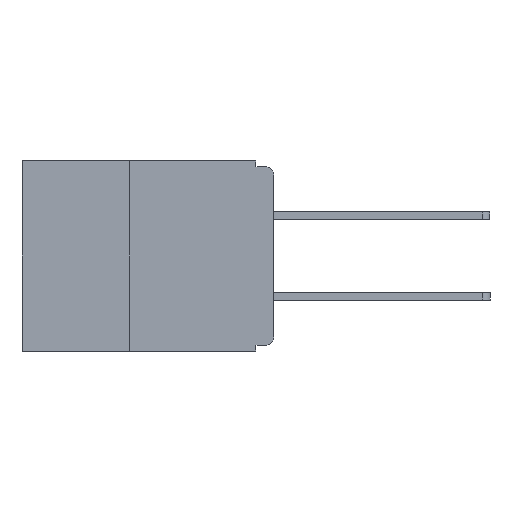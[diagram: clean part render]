
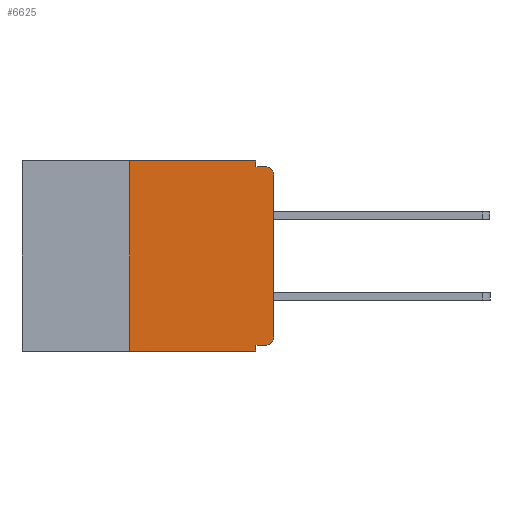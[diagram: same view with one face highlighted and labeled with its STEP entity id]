
A CAD part, left-side view. The second image highlights one B-rep face of the part: STEP entity #6625.
In plain terms, the highlighted planar face has unit normal (-1, 0, 0).
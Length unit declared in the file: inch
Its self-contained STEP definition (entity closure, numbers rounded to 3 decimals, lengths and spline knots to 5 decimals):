
#55 = VERTEX_POINT ( 'NONE', #28646 ) ;
#768 = CIRCLE ( 'NONE', #29298, 0.015 ) ;
#797 = VERTEX_POINT ( 'NONE', #12982 ) ;
#1027 = VERTEX_POINT ( 'NONE', #7774 ) ;
#1044 = CARTESIAN_POINT ( 'NONE',  ( 0., 0., -0.305 ) ) ;
#1522 = VERTEX_POINT ( 'NONE', #11934 ) ;
#2171 = ORIENTED_EDGE ( 'NONE', *, *, #8402, .F. ) ;
#2189 = EDGE_CURVE ( 'NONE', #13385, #2353, #28413, .T. ) ;
#2353 = VERTEX_POINT ( 'NONE', #18320 ) ;
#2566 = EDGE_CURVE ( 'NONE', #1027, #2353, #13446, .T. ) ;
#2572 = CARTESIAN_POINT ( 'NONE',  ( 0., 0.031, 0. ) ) ;
#3139 = CARTESIAN_POINT ( 'NONE',  ( 0., 0.437, 0. ) ) ;
#3473 = VECTOR ( 'NONE', #23259, 39.37008 ) ;
#3894 = ORIENTED_EDGE ( 'NONE', *, *, #29182, .F. ) ;
#4364 = CARTESIAN_POINT ( 'NONE',  ( 0., 0.437, -0.33 ) ) ;
#4496 = DIRECTION ( 'NONE',  ( 0., -1., 0. ) ) ;
#5229 = EDGE_CURVE ( 'NONE', #1522, #14036, #5631, .T. ) ;
#5631 = LINE ( 'NONE', #3139, #28974 ) ;
#6399 = EDGE_CURVE ( 'NONE', #1027, #1522, #10724, .T. ) ;
#6476 = DIRECTION ( 'NONE',  ( -1., 0., 0. ) ) ;
#6625 = ADVANCED_FACE ( 'NONE', ( #10335 ), #24892, .F. ) ;
#6678 = CARTESIAN_POINT ( 'NONE',  ( 0., 0.031, 0. ) ) ;
#7363 = EDGE_LOOP ( 'NONE', ( #29333, #20917, #2171, #3894, #30257, #23526, #18733, #17245, #11721, #22951 ) ) ;
#7774 = CARTESIAN_POINT ( 'NONE',  ( 0., 0.25, -0.33 ) ) ;
#8232 = CARTESIAN_POINT ( 'NONE',  ( 0., 0., -0.025 ) ) ;
#8402 = EDGE_CURVE ( 'NONE', #797, #17838, #15678, .T. ) ;
#10082 = CARTESIAN_POINT ( 'NONE',  ( 0., 0.25, -0.33 ) ) ;
#10335 = FACE_OUTER_BOUND ( 'NONE', #7363, .T. ) ;
#10724 = LINE ( 'NONE', #10082, #22413 ) ;
#10884 = DIRECTION ( 'NONE',  ( 1., 0., 0. ) ) ;
#11721 = ORIENTED_EDGE ( 'NONE', *, *, #17104, .F. ) ;
#11934 = CARTESIAN_POINT ( 'NONE',  ( 0., 0.25, 0. ) ) ;
#11983 = VECTOR ( 'NONE', #4496, 39.37008 ) ;
#12729 = LINE ( 'NONE', #29371, #25201 ) ;
#12819 = CARTESIAN_POINT ( 'NONE',  ( 0., 0., -0.01 ) ) ;
#12982 = CARTESIAN_POINT ( 'NONE',  ( 0., 0.031, -0.01 ) ) ;
#13123 = CARTESIAN_POINT ( 'NONE',  ( 0., 0.437, 0. ) ) ;
#13385 = VERTEX_POINT ( 'NONE', #13543 ) ;
#13446 = LINE ( 'NONE', #4364, #11983 ) ;
#13543 = CARTESIAN_POINT ( 'NONE',  ( 0., 0.031, -0.32 ) ) ;
#14036 = VERTEX_POINT ( 'NONE', #6678 ) ;
#14092 = LINE ( 'NONE', #2572, #19574 ) ;
#14286 = DIRECTION ( 'NONE',  ( -1., 0., 0. ) ) ;
#15057 = EDGE_CURVE ( 'NONE', #26116, #28625, #12729, .T. ) ;
#15372 = CIRCLE ( 'NONE', #20416, 0.015 ) ;
#15678 = LINE ( 'NONE', #12819, #21193 ) ;
#16246 = VECTOR ( 'NONE', #23124, 39.37008 ) ;
#16704 = DIRECTION ( 'NONE',  ( 0., 0., -1. ) ) ;
#17104 = EDGE_CURVE ( 'NONE', #55, #13385, #29343, .T. ) ;
#17240 = DIRECTION ( 'NONE',  ( 0., -1., 0. ) ) ;
#17245 = ORIENTED_EDGE ( 'NONE', *, *, #2189, .F. ) ;
#17838 = VERTEX_POINT ( 'NONE', #19719 ) ;
#18286 = DIRECTION ( 'NONE',  ( 0., 0., -1. ) ) ;
#18320 = CARTESIAN_POINT ( 'NONE',  ( 0., 0.031, -0.33 ) ) ;
#18733 = ORIENTED_EDGE ( 'NONE', *, *, #2566, .T. ) ;
#19355 = DIRECTION ( 'NONE',  ( 0., 0., 1. ) ) ;
#19574 = VECTOR ( 'NONE', #16704, 39.37008 ) ;
#19719 = CARTESIAN_POINT ( 'NONE',  ( 0., 0.015, -0.01 ) ) ;
#19872 = DIRECTION ( 'NONE',  ( 0., -1., 0. ) ) ;
#20090 = EDGE_CURVE ( 'NONE', #55, #26116, #15372, .T. ) ;
#20152 = AXIS2_PLACEMENT_3D ( 'NONE', #13123, #10884, #27239 ) ;
#20416 = AXIS2_PLACEMENT_3D ( 'NONE', #28254, #14286, #18286 ) ;
#20467 = CARTESIAN_POINT ( 'NONE',  ( 0., 0.015, -0.025 ) ) ;
#20742 = CARTESIAN_POINT ( 'NONE',  ( 0., 0., -0.32 ) ) ;
#20917 = ORIENTED_EDGE ( 'NONE', *, *, #26862, .T. ) ;
#21193 = VECTOR ( 'NONE', #19872, 39.37008 ) ;
#22413 = VECTOR ( 'NONE', #19355, 39.37008 ) ;
#22846 = DIRECTION ( 'NONE',  ( 0., 0., -1. ) ) ;
#22951 = ORIENTED_EDGE ( 'NONE', *, *, #20090, .T. ) ;
#23124 = DIRECTION ( 'NONE',  ( 0., 1., 0. ) ) ;
#23259 = DIRECTION ( 'NONE',  ( 0., 0., -1. ) ) ;
#23350 = CARTESIAN_POINT ( 'NONE',  ( 0., 0.031, -0.33 ) ) ;
#23526 = ORIENTED_EDGE ( 'NONE', *, *, #6399, .F. ) ;
#24751 = DIRECTION ( 'NONE',  ( 0., 0., 1. ) ) ;
#24892 = PLANE ( 'NONE',  #20152 ) ;
#25201 = VECTOR ( 'NONE', #24751, 39.37008 ) ;
#26116 = VERTEX_POINT ( 'NONE', #1044 ) ;
#26862 = EDGE_CURVE ( 'NONE', #28625, #17838, #768, .T. ) ;
#27239 = DIRECTION ( 'NONE',  ( 0., 0., -1. ) ) ;
#28254 = CARTESIAN_POINT ( 'NONE',  ( 0., 0.015, -0.305 ) ) ;
#28413 = LINE ( 'NONE', #23350, #3473 ) ;
#28625 = VERTEX_POINT ( 'NONE', #8232 ) ;
#28646 = CARTESIAN_POINT ( 'NONE',  ( 0., 0.015, -0.32 ) ) ;
#28974 = VECTOR ( 'NONE', #17240, 39.37008 ) ;
#29182 = EDGE_CURVE ( 'NONE', #14036, #797, #14092, .T. ) ;
#29298 = AXIS2_PLACEMENT_3D ( 'NONE', #20467, #6476, #22846 ) ;
#29333 = ORIENTED_EDGE ( 'NONE', *, *, #15057, .T. ) ;
#29343 = LINE ( 'NONE', #20742, #16246 ) ;
#29371 = CARTESIAN_POINT ( 'NONE',  ( 0., 0., 0. ) ) ;
#30257 = ORIENTED_EDGE ( 'NONE', *, *, #5229, .F. ) ;
